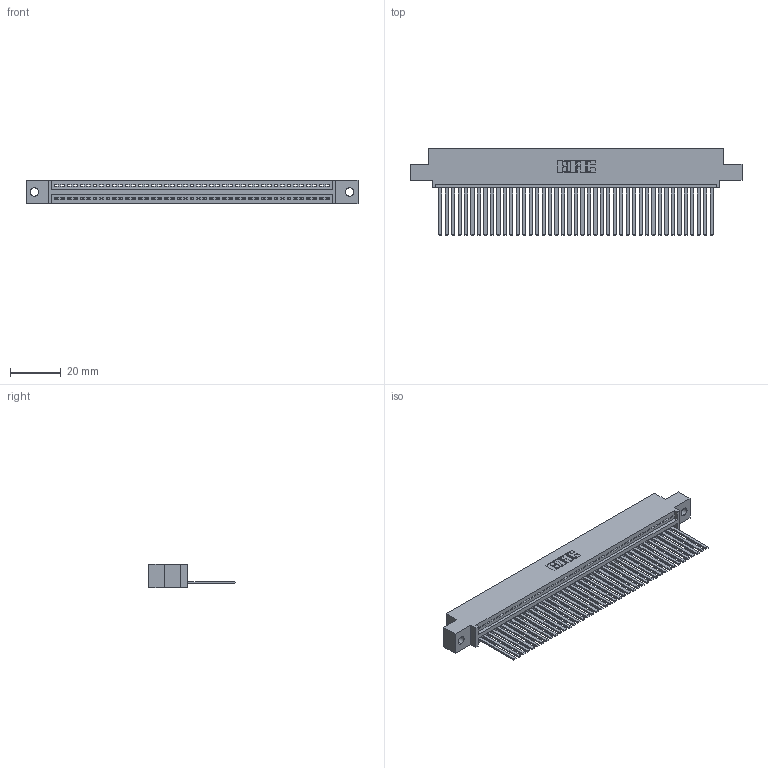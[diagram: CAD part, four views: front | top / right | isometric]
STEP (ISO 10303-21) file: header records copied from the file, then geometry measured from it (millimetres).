
FILE_DESCRIPTION (( 'STEP AP203' ), '1' );
FILE_NAME ('395-043-544-402.STEP', '2018-11-15T16:36:53', ( '' ), ( '' ), 'SwSTEP 2.0', 'SolidWorks 2016', '' );
FILE_SCHEMA (( 'CONFIG_CONTROL_DESIGN' ));
Length unit declared in the file: inch
Products named in the file (3): 345 Part_0.110 Offset - 0.128 Dia; 395-043-544-402; 345-292-001_345-293-144
Assembly tree (44 placements, depth 2):
  395-043-544-402
    345 Part_0.110 Offset - 0.128 Dia
    345-292-001_345-293-144  x43
Bounding box: 130.43 x 33.96 x 9.4 mm (x, y, z)
Volume: 12784.4 mm3; surface area: 18308.3 mm2
Topology: 44 solids, 44 shells, 2366 faces, 7147 edges, 4706 vertices
Faces by surface type: plane 1632, cylinder 734
Entity records: 32179 total; most frequent: CARTESIAN_POINT 5581, ORIENTED_EDGE 5558, DIRECTION 4869, EDGE_CURVE 2779, VECTOR 2479, LINE 2479, VERTEX_POINT 1850, AXIS2_PLACEMENT_3D 1195
